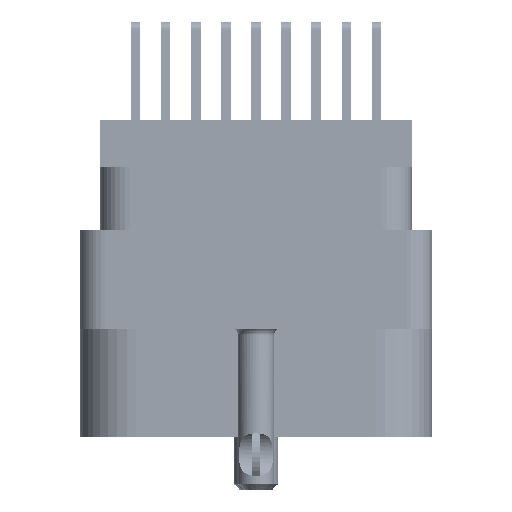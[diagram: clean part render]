
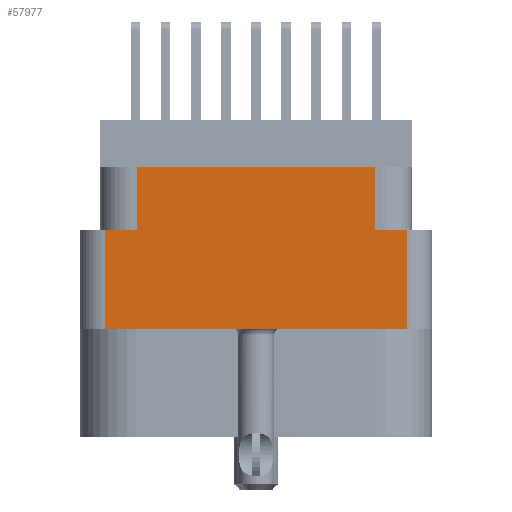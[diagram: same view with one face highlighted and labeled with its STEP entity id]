
A CAD part, left-side view. The second image highlights one B-rep face of the part: STEP entity #57977.
In plain terms, the highlighted planar face has unit normal (-1, 0, 0).
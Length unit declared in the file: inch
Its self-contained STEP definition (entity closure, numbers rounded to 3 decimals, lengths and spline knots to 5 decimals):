
#1011 = CARTESIAN_POINT ( 'NONE',  ( -1.2955, 0.376, -0.789 ) ) ;
#1128 = VECTOR ( 'NONE', #56688, 39.37008 ) ;
#1172 = DIRECTION ( 'NONE',  ( 0., 0., 1. ) ) ;
#1274 = EDGE_CURVE ( 'NONE', #23229, #55007, #25897, .T. ) ;
#3133 = CARTESIAN_POINT ( 'NONE',  ( -1.2955, -0.296, -0.274 ) ) ;
#4326 = CARTESIAN_POINT ( 'NONE',  ( -1.2955, -0.376, -0.274 ) ) ;
#6031 = CARTESIAN_POINT ( 'NONE',  ( -1.2955, 0., -0.274 ) ) ;
#6778 = DIRECTION ( 'NONE',  ( 0., 0., 1. ) ) ;
#7104 = EDGE_CURVE ( 'NONE', #8198, #17530, #39630, .T. ) ;
#7662 = VECTOR ( 'NONE', #1172, 39.37008 ) ;
#8198 = VERTEX_POINT ( 'NONE', #16682 ) ;
#8738 = CARTESIAN_POINT ( 'NONE',  ( -1.2955, -0.296, -0.274 ) ) ;
#9358 = CARTESIAN_POINT ( 'NONE',  ( -1.2955, 0.438, -0.117 ) ) ;
#10965 = CARTESIAN_POINT ( 'NONE',  ( -1.2955, 0., -0.52 ) ) ;
#11600 = VECTOR ( 'NONE', #42345, 39.37008 ) ;
#12952 = CARTESIAN_POINT ( 'NONE',  ( -1.2955, 0.296, -0.117 ) ) ;
#14344 = CARTESIAN_POINT ( 'NONE',  ( -1.2955, 0., -0.274 ) ) ;
#14795 = EDGE_CURVE ( 'NONE', #23229, #30773, #27928, .T. ) ;
#14798 = ORIENTED_EDGE ( 'NONE', *, *, #1274, .F. ) ;
#14911 = VERTEX_POINT ( 'NONE', #22513 ) ;
#14955 = EDGE_CURVE ( 'NONE', #14911, #8198, #23620, .T. ) ;
#16682 = CARTESIAN_POINT ( 'NONE',  ( -1.2955, 0.296, -0.274 ) ) ;
#17430 = ORIENTED_EDGE ( 'NONE', *, *, #7104, .F. ) ;
#17469 = VECTOR ( 'NONE', #39278, 39.37008 ) ;
#17530 = VERTEX_POINT ( 'NONE', #12952 ) ;
#17969 = ORIENTED_EDGE ( 'NONE', *, *, #32142, .F. ) ;
#18747 = ORIENTED_EDGE ( 'NONE', *, *, #38651, .T. ) ;
#20096 = ORIENTED_EDGE ( 'NONE', *, *, #14955, .F. ) ;
#22513 = CARTESIAN_POINT ( 'NONE',  ( -1.2955, 0.376, -0.274 ) ) ;
#22898 = AXIS2_PLACEMENT_3D ( 'NONE', #33991, #56634, #6778 ) ;
#23229 = VERTEX_POINT ( 'NONE', #30024 ) ;
#23294 = ORIENTED_EDGE ( 'NONE', *, *, #14795, .T. ) ;
#23620 = LINE ( 'NONE', #14344, #49302 ) ;
#25897 = LINE ( 'NONE', #10965, #1128 ) ;
#26524 = LINE ( 'NONE', #6031, #11600 ) ;
#27928 = LINE ( 'NONE', #51559, #55001 ) ;
#28690 = CARTESIAN_POINT ( 'NONE',  ( -1.2955, 0.376, -0.52 ) ) ;
#30024 = CARTESIAN_POINT ( 'NONE',  ( -1.2955, -0.376, -0.52 ) ) ;
#30773 = VERTEX_POINT ( 'NONE', #4326 ) ;
#32078 = EDGE_LOOP ( 'NONE', ( #20096, #42705, #14798, #23294, #52717, #18747, #17969, #17430 ) ) ;
#32142 = EDGE_CURVE ( 'NONE', #17530, #57748, #55208, .T. ) ;
#32777 = DIRECTION ( 'NONE',  ( 0., -1., 0. ) ) ;
#33991 = CARTESIAN_POINT ( 'NONE',  ( -1.2955, -0.438, -0.789 ) ) ;
#35418 = EDGE_CURVE ( 'NONE', #14911, #55007, #49241, .T. ) ;
#36552 = DIRECTION ( 'NONE',  ( 0., 0., -1. ) ) ;
#38651 = EDGE_CURVE ( 'NONE', #41672, #57748, #49520, .T. ) ;
#39278 = DIRECTION ( 'NONE',  ( 0., 0., 1. ) ) ;
#39630 = LINE ( 'NONE', #55608, #7662 ) ;
#41272 = EDGE_CURVE ( 'NONE', #41672, #30773, #26524, .T. ) ;
#41672 = VERTEX_POINT ( 'NONE', #8738 ) ;
#42345 = DIRECTION ( 'NONE',  ( 0., -1., 0. ) ) ;
#42705 = ORIENTED_EDGE ( 'NONE', *, *, #35418, .T. ) ;
#43088 = VECTOR ( 'NONE', #32777, 39.37008 ) ;
#44620 = CARTESIAN_POINT ( 'NONE',  ( -1.2955, -0.296, -0.117 ) ) ;
#49241 = LINE ( 'NONE', #1011, #54267 ) ;
#49302 = VECTOR ( 'NONE', #51137, 39.37008 ) ;
#49520 = LINE ( 'NONE', #3133, #17469 ) ;
#51137 = DIRECTION ( 'NONE',  ( 0., -1., 0. ) ) ;
#51375 = DIRECTION ( 'NONE',  ( 0., 0., 1. ) ) ;
#51559 = CARTESIAN_POINT ( 'NONE',  ( -1.2955, -0.376, -0.789 ) ) ;
#52055 = PLANE ( 'NONE',  #22898 ) ;
#52717 = ORIENTED_EDGE ( 'NONE', *, *, #41272, .F. ) ;
#54267 = VECTOR ( 'NONE', #36552, 39.37008 ) ;
#55001 = VECTOR ( 'NONE', #51375, 39.37008 ) ;
#55007 = VERTEX_POINT ( 'NONE', #28690 ) ;
#55208 = LINE ( 'NONE', #9358, #43088 ) ;
#55608 = CARTESIAN_POINT ( 'NONE',  ( -1.2955, 0.296, -0.274 ) ) ;
#56634 = DIRECTION ( 'NONE',  ( -1., 0., 0. ) ) ;
#56688 = DIRECTION ( 'NONE',  ( 0., 1., 0. ) ) ;
#57748 = VERTEX_POINT ( 'NONE', #44620 ) ;
#57937 = FACE_OUTER_BOUND ( 'NONE', #32078, .T. ) ;
#57977 = ADVANCED_FACE ( 'NONE', ( #57937 ), #52055, .T. ) ;
